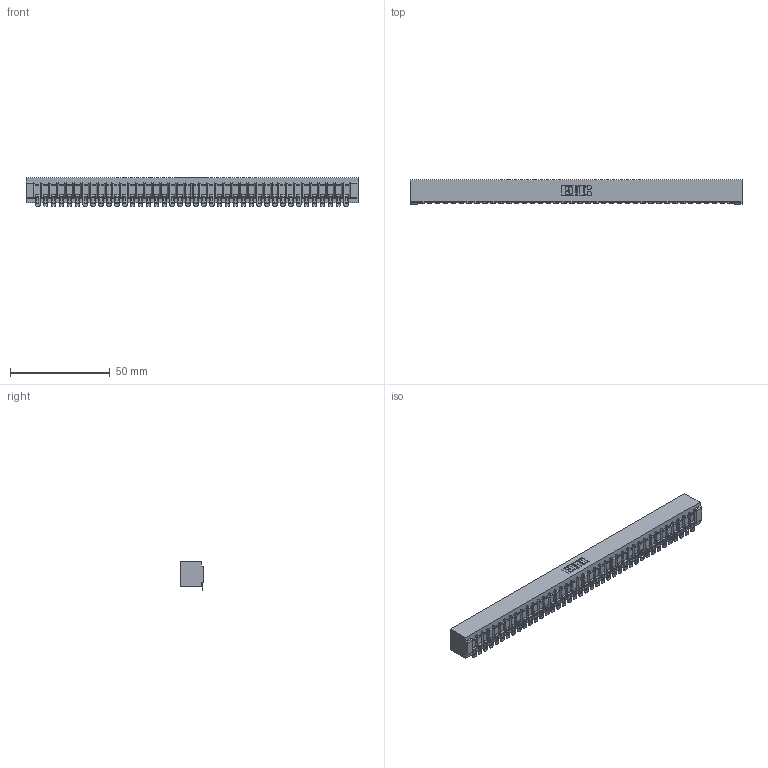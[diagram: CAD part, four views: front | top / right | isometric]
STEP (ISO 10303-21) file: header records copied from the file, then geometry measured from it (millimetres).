
FILE_DESCRIPTION (( 'STEP AP203' ), '1' );
FILE_NAME ('357-040-554-101.STEP', '2019-09-17T09:13:51', ( '' ), ( '' ), 'SwSTEP 2.0', 'SolidWorks 2016', '' );
FILE_SCHEMA (( 'CONFIG_CONTROL_DESIGN' ));
Length unit declared in the file: inch
Products named in the file (3): 357-040-554-101; 307 Part_No Mounting Lugs; 307-290-002_554
Assembly tree (41 placements, depth 2):
  357-040-554-101
    307 Part_No Mounting Lugs
    307-290-002_554  x40
Bounding box: 166.37 x 12.01 x 14.52 mm (x, y, z)
Volume: 18360.9 mm3; surface area: 23546.1 mm2
Topology: 41 solids, 41 shells, 3391 faces, 10419 edges, 6834 vertices
Faces by surface type: plane 1906, cylinder 1403, sphere 82
Entity records: 35225 total; most frequent: CARTESIAN_POINT 5942, ORIENTED_EDGE 5932, DIRECTION 5778, EDGE_CURVE 2966, VECTOR 2266, LINE 2266, VERTEX_POINT 1920, AXIS2_PLACEMENT_3D 1756
